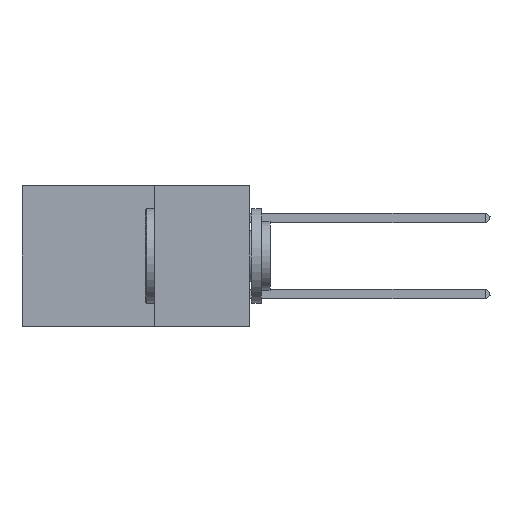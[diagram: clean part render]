
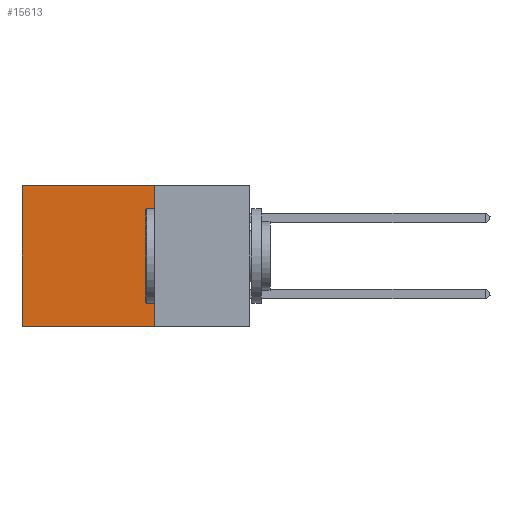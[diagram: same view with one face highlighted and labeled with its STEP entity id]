
A CAD part, left-side view. The second image highlights one B-rep face of the part: STEP entity #15613.
In plain terms, the highlighted planar face has unit normal (-1, 0, 0).
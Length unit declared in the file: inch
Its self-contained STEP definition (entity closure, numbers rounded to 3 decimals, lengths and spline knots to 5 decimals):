
#691 = ORIENTED_EDGE ( 'NONE', *, *, #29318, .F. ) ;
#868 = LINE ( 'NONE', #29029, #27903 ) ;
#1067 = FACE_OUTER_BOUND ( 'NONE', #4329, .T. ) ;
#1964 = VECTOR ( 'NONE', #15941, 39.37008 ) ;
#3314 = DIRECTION ( 'NONE',  ( 1., 0., 0. ) ) ;
#4177 = VECTOR ( 'NONE', #7731, 39.37008 ) ;
#4329 = EDGE_LOOP ( 'NONE', ( #32146, #691, #12842, #39589 ) ) ;
#6040 = DIRECTION ( 'NONE',  ( 0., 1., 0. ) ) ;
#6645 = DIRECTION ( 'NONE',  ( 0., 0., -1. ) ) ;
#7720 = VERTEX_POINT ( 'NONE', #41312 ) ;
#7731 = DIRECTION ( 'NONE',  ( 0., 0., -1. ) ) ;
#11138 = LINE ( 'NONE', #26220, #1964 ) ;
#12345 = VERTEX_POINT ( 'NONE', #37230 ) ;
#12842 = ORIENTED_EDGE ( 'NONE', *, *, #17187, .F. ) ;
#15613 = ADVANCED_FACE ( 'NONE', ( #1067 ), #17378, .F. ) ;
#15941 = DIRECTION ( 'NONE',  ( 0., 1., 0. ) ) ;
#17187 = EDGE_CURVE ( 'NONE', #12345, #24585, #40973, .T. ) ;
#17378 = PLANE ( 'NONE',  #21913 ) ;
#18398 = VERTEX_POINT ( 'NONE', #42207 ) ;
#18404 = DIRECTION ( 'NONE',  ( 0., 0., -1. ) ) ;
#18760 = EDGE_CURVE ( 'NONE', #12345, #18398, #11138, .T. ) ;
#21913 = AXIS2_PLACEMENT_3D ( 'NONE', #37776, #3314, #6645 ) ;
#24585 = VERTEX_POINT ( 'NONE', #41773 ) ;
#26181 = EDGE_CURVE ( 'NONE', #18398, #7720, #868, .T. ) ;
#26220 = CARTESIAN_POINT ( 'NONE',  ( 0.2875, 0.25, 0. ) ) ;
#26827 = VECTOR ( 'NONE', #6040, 39.37008 ) ;
#27903 = VECTOR ( 'NONE', #18404, 39.37008 ) ;
#29029 = CARTESIAN_POINT ( 'NONE',  ( 0.2875, 0.6, 0. ) ) ;
#29318 = EDGE_CURVE ( 'NONE', #24585, #7720, #34922, .T. ) ;
#32146 = ORIENTED_EDGE ( 'NONE', *, *, #26181, .T. ) ;
#34922 = LINE ( 'NONE', #44548, #26827 ) ;
#35406 = CARTESIAN_POINT ( 'NONE',  ( 0.2875, 0.25, 0. ) ) ;
#37230 = CARTESIAN_POINT ( 'NONE',  ( 0.2875, 0.25, 0. ) ) ;
#37776 = CARTESIAN_POINT ( 'NONE',  ( 0.2875, 0.25, 0. ) ) ;
#39589 = ORIENTED_EDGE ( 'NONE', *, *, #18760, .T. ) ;
#40973 = LINE ( 'NONE', #35406, #4177 ) ;
#41312 = CARTESIAN_POINT ( 'NONE',  ( 0.2875, 0.6, -0.37 ) ) ;
#41773 = CARTESIAN_POINT ( 'NONE',  ( 0.2875, 0.25, -0.37 ) ) ;
#42207 = CARTESIAN_POINT ( 'NONE',  ( 0.2875, 0.6, 0. ) ) ;
#44548 = CARTESIAN_POINT ( 'NONE',  ( 0.2875, 0.25, -0.37 ) ) ;
